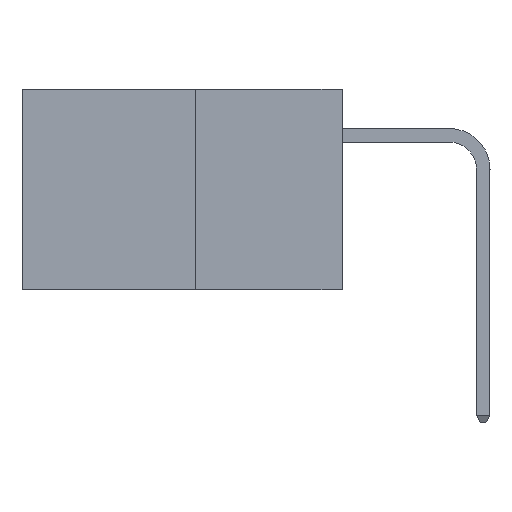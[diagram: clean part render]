
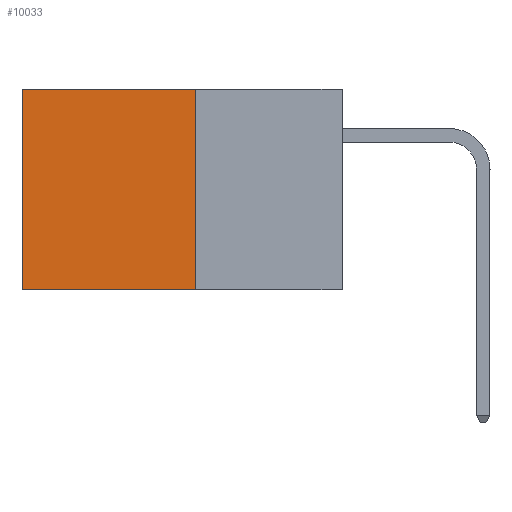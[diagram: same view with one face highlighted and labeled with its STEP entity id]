
A CAD part, left-side view. The second image highlights one B-rep face of the part: STEP entity #10033.
In plain terms, the highlighted planar face has unit normal (-1, 0, 0).
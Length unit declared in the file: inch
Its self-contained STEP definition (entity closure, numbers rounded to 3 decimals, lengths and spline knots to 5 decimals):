
#364 = LINE ( 'NONE', #9271, #3652 ) ;
#460 = CARTESIAN_POINT ( 'NONE',  ( 0.277, 0.59, 0. ) ) ;
#942 = CARTESIAN_POINT ( 'NONE',  ( 0.277, 0.59, -0.37 ) ) ;
#1819 = ORIENTED_EDGE ( 'NONE', *, *, #5716, .T. ) ;
#2178 = ORIENTED_EDGE ( 'NONE', *, *, #9940, .F. ) ;
#2353 = DIRECTION ( 'NONE',  ( 0., 0., -1. ) ) ;
#2502 = DIRECTION ( 'NONE',  ( 1., 0., 0. ) ) ;
#2642 = EDGE_LOOP ( 'NONE', ( #1819, #7942, #2178, #5214 ) ) ;
#3652 = VECTOR ( 'NONE', #2353, 39.37008 ) ;
#3670 = CARTESIAN_POINT ( 'NONE',  ( 0.277, 0.27, -0.37 ) ) ;
#4005 = EDGE_CURVE ( 'NONE', #4780, #10573, #12927, .T. ) ;
#4018 = VECTOR ( 'NONE', #14638, 39.37008 ) ;
#4522 = DIRECTION ( 'NONE',  ( 0., 0., -1. ) ) ;
#4780 = VERTEX_POINT ( 'NONE', #3670 ) ;
#5002 = CARTESIAN_POINT ( 'NONE',  ( 0.277, 0.27, 0. ) ) ;
#5214 = ORIENTED_EDGE ( 'NONE', *, *, #13233, .T. ) ;
#5716 = EDGE_CURVE ( 'NONE', #12409, #10573, #7772, .T. ) ;
#7772 = LINE ( 'NONE', #10334, #13602 ) ;
#7942 = ORIENTED_EDGE ( 'NONE', *, *, #4005, .F. ) ;
#8132 = CARTESIAN_POINT ( 'NONE',  ( 0.277, 0.27, 0. ) ) ;
#8189 = LINE ( 'NONE', #5002, #14004 ) ;
#8356 = FACE_OUTER_BOUND ( 'NONE', #2642, .T. ) ;
#9271 = CARTESIAN_POINT ( 'NONE',  ( 0.277, 0.27, -0.37 ) ) ;
#9432 = CARTESIAN_POINT ( 'NONE',  ( 0.277, 0.27, -0.37 ) ) ;
#9940 = EDGE_CURVE ( 'NONE', #12811, #4780, #364, .T. ) ;
#10033 = ADVANCED_FACE ( 'NONE', ( #8356 ), #15175, .F. ) ;
#10334 = CARTESIAN_POINT ( 'NONE',  ( 0.277, 0.59, -0.37 ) ) ;
#10573 = VERTEX_POINT ( 'NONE', #942 ) ;
#10588 = DIRECTION ( 'NONE',  ( 0., 0., -1. ) ) ;
#11435 = AXIS2_PLACEMENT_3D ( 'NONE', #9432, #2502, #10588 ) ;
#12039 = DIRECTION ( 'NONE',  ( 0., 1., 0. ) ) ;
#12409 = VERTEX_POINT ( 'NONE', #460 ) ;
#12811 = VERTEX_POINT ( 'NONE', #8132 ) ;
#12927 = LINE ( 'NONE', #14646, #4018 ) ;
#13233 = EDGE_CURVE ( 'NONE', #12811, #12409, #8189, .T. ) ;
#13602 = VECTOR ( 'NONE', #4522, 39.37008 ) ;
#14004 = VECTOR ( 'NONE', #12039, 39.37008 ) ;
#14638 = DIRECTION ( 'NONE',  ( 0., 1., 0. ) ) ;
#14646 = CARTESIAN_POINT ( 'NONE',  ( 0.277, 0.27, -0.37 ) ) ;
#15175 = PLANE ( 'NONE',  #11435 ) ;
